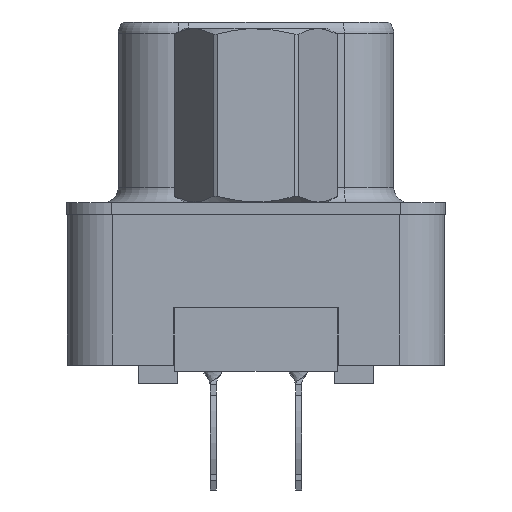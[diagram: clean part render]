
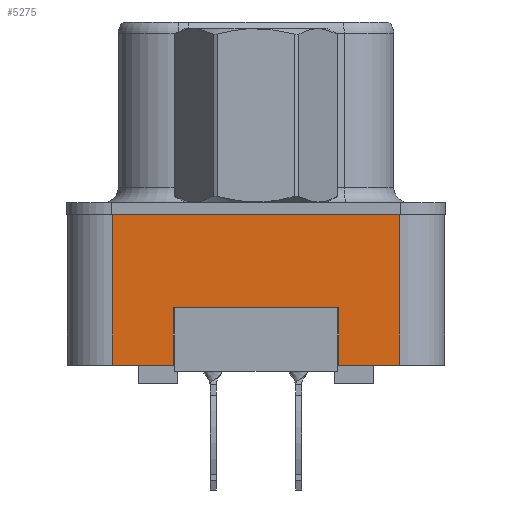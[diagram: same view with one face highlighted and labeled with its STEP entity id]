
A CAD part, left-side view. The second image highlights one B-rep face of the part: STEP entity #5275.
In plain terms, the highlighted planar face has unit normal (-1, 0, 0).
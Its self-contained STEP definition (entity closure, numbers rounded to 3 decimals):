
#664 = LINE ( 'NONE', #16174, #8844 ) ;
#813 = VERTEX_POINT ( 'NONE', #22066 ) ;
#977 = VECTOR ( 'NONE', #2391, 1000. ) ;
#1013 = DIRECTION ( 'NONE',  ( -1., 0., 0. ) ) ;
#1647 = AXIS2_PLACEMENT_3D ( 'NONE', #26451, #1013, #16961 ) ;
#2391 = DIRECTION ( 'NONE',  ( 0., 0., -1. ) ) ;
#3206 = CARTESIAN_POINT ( 'NONE',  ( -3., -2.75, -3.1 ) ) ;
#3692 = LINE ( 'NONE', #7918, #7966 ) ;
#4328 = ORIENTED_EDGE ( 'NONE', *, *, #27464, .T. ) ;
#4743 = DIRECTION ( 'NONE',  ( 0., 0., 1. ) ) ;
#4983 = EDGE_CURVE ( 'NONE', #813, #25037, #13557, .T. ) ;
#5275 = ADVANCED_FACE ( 'NONE', ( #28446 ), #7803, .T. ) ;
#5293 = ORIENTED_EDGE ( 'NONE', *, *, #13577, .T. ) ;
#6676 = ORIENTED_EDGE ( 'NONE', *, *, #18342, .F. ) ;
#7803 = PLANE ( 'NONE',  #1647 ) ;
#7900 = VECTOR ( 'NONE', #12363, 1000. ) ;
#7918 = CARTESIAN_POINT ( 'NONE',  ( -3., -4.775, 0. ) ) ;
#7966 = VECTOR ( 'NONE', #26277, 1000. ) ;
#8600 = VERTEX_POINT ( 'NONE', #9420 ) ;
#8693 = ORIENTED_EDGE ( 'NONE', *, *, #12838, .F. ) ;
#8765 = CARTESIAN_POINT ( 'NONE',  ( -3., -4.775, -5. ) ) ;
#8778 = EDGE_CURVE ( 'NONE', #23825, #8600, #23847, .T. ) ;
#8844 = VECTOR ( 'NONE', #4743, 1000. ) ;
#9420 = CARTESIAN_POINT ( 'NONE',  ( -3., -2.75, -5. ) ) ;
#9424 = ORIENTED_EDGE ( 'NONE', *, *, #4983, .T. ) ;
#9541 = LINE ( 'NONE', #9836, #13188 ) ;
#9836 = CARTESIAN_POINT ( 'NONE',  ( -3., -4.775, -5. ) ) ;
#9853 = DIRECTION ( 'NONE',  ( 0., 0., -1. ) ) ;
#9915 = CARTESIAN_POINT ( 'NONE',  ( -3., 2.75, -3.1 ) ) ;
#11112 = EDGE_CURVE ( 'NONE', #11239, #25037, #3692, .T. ) ;
#11239 = VERTEX_POINT ( 'NONE', #24761 ) ;
#11590 = ORIENTED_EDGE ( 'NONE', *, *, #14443, .F. ) ;
#11643 = VECTOR ( 'NONE', #25496, 1000. ) ;
#12213 = LINE ( 'NONE', #16854, #7900 ) ;
#12363 = DIRECTION ( 'NONE',  ( 0., -1., 0. ) ) ;
#12838 = EDGE_CURVE ( 'NONE', #19541, #11239, #664, .T. ) ;
#13038 = CARTESIAN_POINT ( 'NONE',  ( -3., -2.75, -3.1 ) ) ;
#13188 = VECTOR ( 'NONE', #18704, 1000. ) ;
#13557 = LINE ( 'NONE', #8765, #14790 ) ;
#13577 = EDGE_CURVE ( 'NONE', #19541, #16390, #12213, .T. ) ;
#14443 = EDGE_CURVE ( 'NONE', #21190, #16390, #18644, .T. ) ;
#14790 = VECTOR ( 'NONE', #22314, 1000. ) ;
#16174 = CARTESIAN_POINT ( 'NONE',  ( -3., 4.775, -5. ) ) ;
#16390 = VERTEX_POINT ( 'NONE', #24325 ) ;
#16502 = EDGE_LOOP ( 'NONE', ( #23041, #4328, #9424, #22523, #8693, #5293, #11590, #6676 ) ) ;
#16854 = CARTESIAN_POINT ( 'NONE',  ( -3., -4.775, -5. ) ) ;
#16961 = DIRECTION ( 'NONE',  ( 0., 0., 1. ) ) ;
#18342 = EDGE_CURVE ( 'NONE', #23825, #21190, #23245, .T. ) ;
#18644 = LINE ( 'NONE', #9915, #977 ) ;
#18704 = DIRECTION ( 'NONE',  ( 0., -1., 0. ) ) ;
#19541 = VERTEX_POINT ( 'NONE', #23249 ) ;
#19799 = CARTESIAN_POINT ( 'NONE',  ( -3., -4.775, 0. ) ) ;
#21190 = VERTEX_POINT ( 'NONE', #23509 ) ;
#22066 = CARTESIAN_POINT ( 'NONE',  ( -3., -4.775, -5. ) ) ;
#22314 = DIRECTION ( 'NONE',  ( 0., 0., 1. ) ) ;
#22523 = ORIENTED_EDGE ( 'NONE', *, *, #11112, .F. ) ;
#23041 = ORIENTED_EDGE ( 'NONE', *, *, #8778, .T. ) ;
#23245 = LINE ( 'NONE', #26063, #11643 ) ;
#23249 = CARTESIAN_POINT ( 'NONE',  ( -3., 4.775, -5. ) ) ;
#23509 = CARTESIAN_POINT ( 'NONE',  ( -3., 2.75, -3.1 ) ) ;
#23825 = VERTEX_POINT ( 'NONE', #13038 ) ;
#23847 = LINE ( 'NONE', #3206, #29314 ) ;
#24325 = CARTESIAN_POINT ( 'NONE',  ( -3., 2.75, -5. ) ) ;
#24761 = CARTESIAN_POINT ( 'NONE',  ( -3., 4.775, 0. ) ) ;
#25037 = VERTEX_POINT ( 'NONE', #19799 ) ;
#25496 = DIRECTION ( 'NONE',  ( 0., 1., 0. ) ) ;
#26063 = CARTESIAN_POINT ( 'NONE',  ( -3., 2.75, -3.1 ) ) ;
#26277 = DIRECTION ( 'NONE',  ( 0., -1., 0. ) ) ;
#26451 = CARTESIAN_POINT ( 'NONE',  ( -3., -4.775, -5. ) ) ;
#27464 = EDGE_CURVE ( 'NONE', #8600, #813, #9541, .T. ) ;
#28446 = FACE_OUTER_BOUND ( 'NONE', #16502, .T. ) ;
#29314 = VECTOR ( 'NONE', #9853, 1000. ) ;
